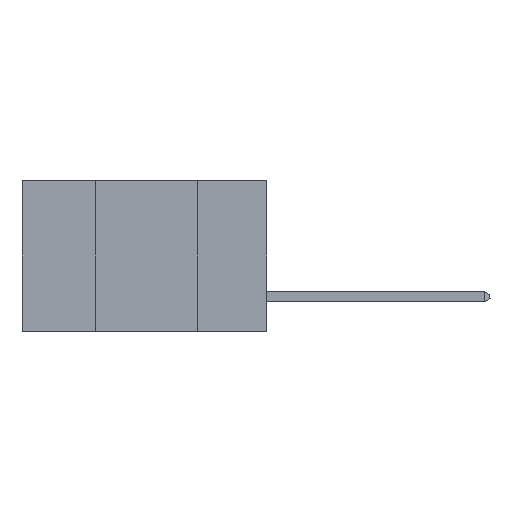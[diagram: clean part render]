
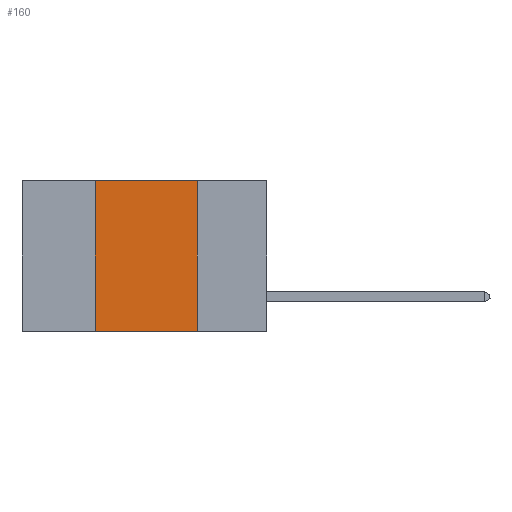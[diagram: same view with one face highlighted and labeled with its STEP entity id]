
A CAD part, left-side view. The second image highlights one B-rep face of the part: STEP entity #160.
In plain terms, the highlighted planar face has unit normal (-1, 0, 0).
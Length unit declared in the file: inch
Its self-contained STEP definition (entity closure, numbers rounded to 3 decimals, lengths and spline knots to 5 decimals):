
#160 = ADVANCED_FACE ( 'NONE', ( #21957 ), #8416, .F. ) ;
#1640 = EDGE_LOOP ( 'NONE', ( #2343, #6347, #16459, #11763 ) ) ;
#1965 = LINE ( 'NONE', #14276, #12557 ) ;
#2038 = VECTOR ( 'NONE', #12518, 39.37008 ) ;
#2089 = DIRECTION ( 'NONE',  ( 0., -1., 0. ) ) ;
#2343 = ORIENTED_EDGE ( 'NONE', *, *, #10240, .F. ) ;
#3296 = VERTEX_POINT ( 'NONE', #20328 ) ;
#5307 = VERTEX_POINT ( 'NONE', #11059 ) ;
#6347 = ORIENTED_EDGE ( 'NONE', *, *, #17532, .F. ) ;
#7470 = CARTESIAN_POINT ( 'NONE',  ( 0., 0.6, 0. ) ) ;
#7764 = LINE ( 'NONE', #7470, #16456 ) ;
#8339 = LINE ( 'NONE', #17338, #12274 ) ;
#8416 = PLANE ( 'NONE',  #8636 ) ;
#8636 = AXIS2_PLACEMENT_3D ( 'NONE', #10203, #20985, #13883 ) ;
#9198 = CARTESIAN_POINT ( 'NONE',  ( 0., 0.42, 0. ) ) ;
#10203 = CARTESIAN_POINT ( 'NONE',  ( 0., 0.6, 0. ) ) ;
#10240 = EDGE_CURVE ( 'NONE', #11498, #5307, #8339, .T. ) ;
#11059 = CARTESIAN_POINT ( 'NONE',  ( 0., 0.17, -0.37 ) ) ;
#11498 = VERTEX_POINT ( 'NONE', #15356 ) ;
#11763 = ORIENTED_EDGE ( 'NONE', *, *, #15152, .T. ) ;
#12063 = DIRECTION ( 'NONE',  ( 0., 0., -1. ) ) ;
#12274 = VECTOR ( 'NONE', #12063, 39.37008 ) ;
#12518 = DIRECTION ( 'NONE',  ( 0., -1., 0. ) ) ;
#12557 = VECTOR ( 'NONE', #19769, 39.37008 ) ;
#13883 = DIRECTION ( 'NONE',  ( 0., 0., -1. ) ) ;
#14276 = CARTESIAN_POINT ( 'NONE',  ( 0., 0.42, 0. ) ) ;
#15152 = EDGE_CURVE ( 'NONE', #3296, #5307, #16280, .T. ) ;
#15356 = CARTESIAN_POINT ( 'NONE',  ( 0., 0.17, 0. ) ) ;
#16059 = CARTESIAN_POINT ( 'NONE',  ( 0., 0.6, -0.37 ) ) ;
#16280 = LINE ( 'NONE', #16059, #2038 ) ;
#16456 = VECTOR ( 'NONE', #2089, 39.37008 ) ;
#16459 = ORIENTED_EDGE ( 'NONE', *, *, #20414, .F. ) ;
#17226 = VERTEX_POINT ( 'NONE', #9198 ) ;
#17338 = CARTESIAN_POINT ( 'NONE',  ( 0., 0.17, 0. ) ) ;
#17532 = EDGE_CURVE ( 'NONE', #17226, #11498, #7764, .T. ) ;
#19769 = DIRECTION ( 'NONE',  ( 0., 0., 1. ) ) ;
#20328 = CARTESIAN_POINT ( 'NONE',  ( 0., 0.42, -0.37 ) ) ;
#20414 = EDGE_CURVE ( 'NONE', #3296, #17226, #1965, .T. ) ;
#20985 = DIRECTION ( 'NONE',  ( 1., 0., 0. ) ) ;
#21957 = FACE_OUTER_BOUND ( 'NONE', #1640, .T. ) ;
